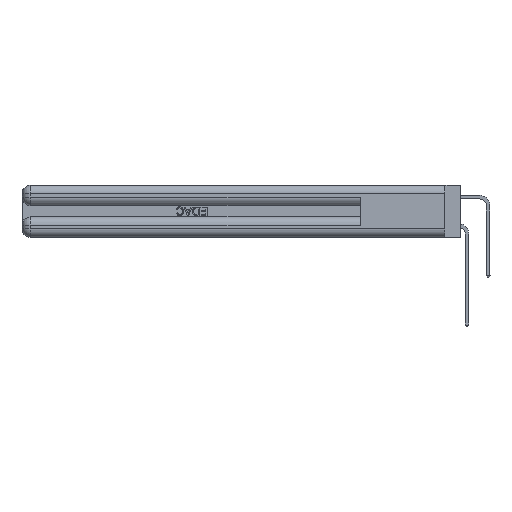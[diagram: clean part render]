
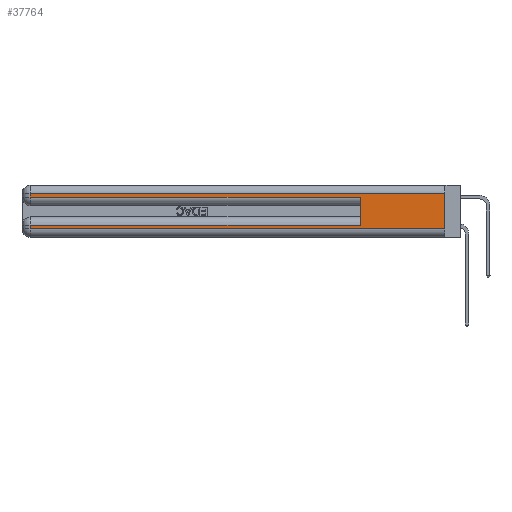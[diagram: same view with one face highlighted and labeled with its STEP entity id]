
A CAD part, left-side view. The second image highlights one B-rep face of the part: STEP entity #37764.
In plain terms, the highlighted planar face has unit normal (-1, 0, 0).
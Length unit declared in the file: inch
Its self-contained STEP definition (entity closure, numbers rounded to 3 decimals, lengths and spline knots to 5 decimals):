
#1541 = EDGE_LOOP ( 'NONE', ( #15565, #4806, #36867, #6775, #45055, #25491, #26782, #20175 ) ) ;
#1564 = EDGE_CURVE ( 'NONE', #18511, #19982, #27696, .T. ) ;
#3814 = CARTESIAN_POINT ( 'NONE',  ( 0., 2.94, 0.085 ) ) ;
#3893 = DIRECTION ( 'NONE',  ( 0., 0., -1. ) ) ;
#4806 = ORIENTED_EDGE ( 'NONE', *, *, #40486, .T. ) ;
#4958 = CARTESIAN_POINT ( 'NONE',  ( 0., 0.6, 0.145 ) ) ;
#5066 = LINE ( 'NONE', #12874, #24175 ) ;
#5091 = EDGE_CURVE ( 'NONE', #25397, #48419, #44152, .T. ) ;
#5251 = CARTESIAN_POINT ( 'NONE',  ( 0., 2.94, 0.285 ) ) ;
#6238 = VERTEX_POINT ( 'NONE', #3814 ) ;
#6775 = ORIENTED_EDGE ( 'NONE', *, *, #1564, .T. ) ;
#7394 = VECTOR ( 'NONE', #29434, 39.37008 ) ;
#7502 = CARTESIAN_POINT ( 'NONE',  ( 0., 0., 0.31 ) ) ;
#8405 = PLANE ( 'NONE',  #19936 ) ;
#8675 = VERTEX_POINT ( 'NONE', #7502 ) ;
#9000 = DIRECTION ( 'NONE',  ( 0., 0., -1. ) ) ;
#11791 = VECTOR ( 'NONE', #39440, 39.37008 ) ;
#12273 = DIRECTION ( 'NONE',  ( 1., 0., 0. ) ) ;
#12874 = CARTESIAN_POINT ( 'NONE',  ( 0., 0., 0.37 ) ) ;
#14006 = VECTOR ( 'NONE', #27278, 39.37008 ) ;
#15565 = ORIENTED_EDGE ( 'NONE', *, *, #34922, .F. ) ;
#18511 = VERTEX_POINT ( 'NONE', #5251 ) ;
#18714 = VERTEX_POINT ( 'NONE', #25463 ) ;
#19936 = AXIS2_PLACEMENT_3D ( 'NONE', #46130, #12273, #38791 ) ;
#19982 = VERTEX_POINT ( 'NONE', #44329 ) ;
#20175 = ORIENTED_EDGE ( 'NONE', *, *, #5091, .T. ) ;
#20567 = CARTESIAN_POINT ( 'NONE',  ( 0., 0.6, 0.085 ) ) ;
#21076 = LINE ( 'NONE', #47058, #39981 ) ;
#21753 = CARTESIAN_POINT ( 'NONE',  ( 0., 0., 0.285 ) ) ;
#22175 = CARTESIAN_POINT ( 'NONE',  ( 0., 2.94, 0.37 ) ) ;
#24175 = VECTOR ( 'NONE', #9000, 39.37008 ) ;
#24377 = EDGE_CURVE ( 'NONE', #32776, #6238, #21076, .T. ) ;
#24426 = CARTESIAN_POINT ( 'NONE',  ( 0., 0., 0.31 ) ) ;
#25397 = VERTEX_POINT ( 'NONE', #31414 ) ;
#25463 = CARTESIAN_POINT ( 'NONE',  ( 0., 2.94, 0.31 ) ) ;
#25491 = ORIENTED_EDGE ( 'NONE', *, *, #24377, .T. ) ;
#26257 = CARTESIAN_POINT ( 'NONE',  ( 0., 0., 0.06 ) ) ;
#26782 = ORIENTED_EDGE ( 'NONE', *, *, #35255, .T. ) ;
#26818 = VECTOR ( 'NONE', #35406, 39.37008 ) ;
#27278 = DIRECTION ( 'NONE',  ( 0., -1., 0. ) ) ;
#27696 = LINE ( 'NONE', #21753, #7394 ) ;
#28556 = DIRECTION ( 'NONE',  ( 0., 1., 0. ) ) ;
#29434 = DIRECTION ( 'NONE',  ( 0., -1., 0. ) ) ;
#29612 = LINE ( 'NONE', #22175, #39566 ) ;
#29948 = FACE_OUTER_BOUND ( 'NONE', #1541, .T. ) ;
#30439 = EDGE_CURVE ( 'NONE', #32776, #19982, #39164, .T. ) ;
#30569 = VECTOR ( 'NONE', #3893, 39.37008 ) ;
#31414 = CARTESIAN_POINT ( 'NONE',  ( 0., 2.94, 0.06 ) ) ;
#31992 = LINE ( 'NONE', #24426, #11791 ) ;
#32776 = VERTEX_POINT ( 'NONE', #20567 ) ;
#34922 = EDGE_CURVE ( 'NONE', #8675, #48419, #5066, .T. ) ;
#35255 = EDGE_CURVE ( 'NONE', #6238, #25397, #29612, .T. ) ;
#35406 = DIRECTION ( 'NONE',  ( 0., 0., 1. ) ) ;
#36867 = ORIENTED_EDGE ( 'NONE', *, *, #42766, .T. ) ;
#37764 = ADVANCED_FACE ( 'NONE', ( #29948 ), #8405, .F. ) ;
#38791 = DIRECTION ( 'NONE',  ( 0., 0., -1. ) ) ;
#39164 = LINE ( 'NONE', #4958, #26818 ) ;
#39440 = DIRECTION ( 'NONE',  ( 0., 1., 0. ) ) ;
#39566 = VECTOR ( 'NONE', #40983, 39.37008 ) ;
#39981 = VECTOR ( 'NONE', #28556, 39.37008 ) ;
#40486 = EDGE_CURVE ( 'NONE', #8675, #18714, #31992, .T. ) ;
#40540 = LINE ( 'NONE', #45335, #30569 ) ;
#40983 = DIRECTION ( 'NONE',  ( 0., 0., -1. ) ) ;
#42214 = CARTESIAN_POINT ( 'NONE',  ( 0., 0., 0.06 ) ) ;
#42766 = EDGE_CURVE ( 'NONE', #18714, #18511, #40540, .T. ) ;
#44152 = LINE ( 'NONE', #42214, #14006 ) ;
#44329 = CARTESIAN_POINT ( 'NONE',  ( 0., 0.6, 0.285 ) ) ;
#45055 = ORIENTED_EDGE ( 'NONE', *, *, #30439, .F. ) ;
#45335 = CARTESIAN_POINT ( 'NONE',  ( 0., 2.94, 0.37 ) ) ;
#46130 = CARTESIAN_POINT ( 'NONE',  ( 0., 0., 0.37 ) ) ;
#47058 = CARTESIAN_POINT ( 'NONE',  ( 0., 0., 0.085 ) ) ;
#48419 = VERTEX_POINT ( 'NONE', #26257 ) ;
